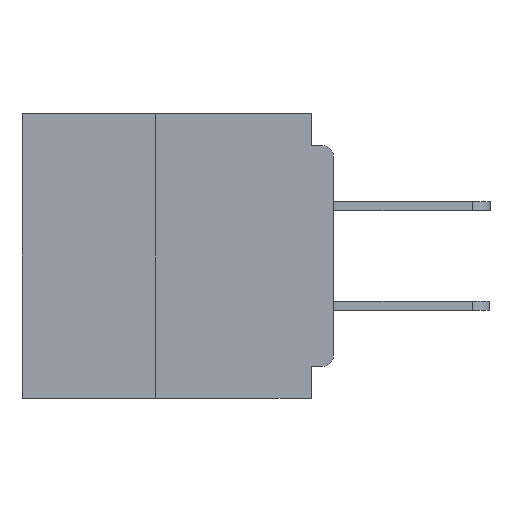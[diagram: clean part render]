
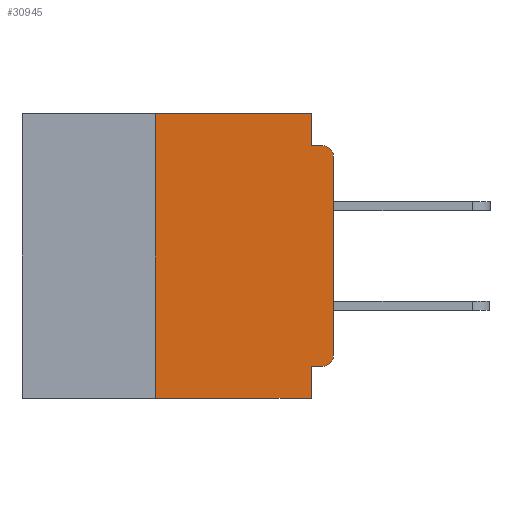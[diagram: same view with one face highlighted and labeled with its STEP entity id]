
A CAD part, left-side view. The second image highlights one B-rep face of the part: STEP entity #30945.
In plain terms, the highlighted planar face has unit normal (-1, 0, 0).
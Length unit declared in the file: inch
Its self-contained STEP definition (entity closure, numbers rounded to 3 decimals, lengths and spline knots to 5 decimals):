
#432 = VERTEX_POINT ( 'NONE', #10456 ) ;
#703 = VECTOR ( 'NONE', #32808, 39.37008 ) ;
#1035 = VECTOR ( 'NONE', #26939, 39.37008 ) ;
#1875 = ORIENTED_EDGE ( 'NONE', *, *, #35211, .T. ) ;
#3511 = ORIENTED_EDGE ( 'NONE', *, *, #10251, .F. ) ;
#3592 = DIRECTION ( 'NONE',  ( 1., 0., 0. ) ) ;
#3890 = LINE ( 'NONE', #31665, #19106 ) ;
#3931 = DIRECTION ( 'NONE',  ( 0., -1., 0. ) ) ;
#4588 = DIRECTION ( 'NONE',  ( 0., 1., 0. ) ) ;
#5513 = AXIS2_PLACEMENT_3D ( 'NONE', #20702, #3592, #23549 ) ;
#5674 = VECTOR ( 'NONE', #4588, 39.37008 ) ;
#6583 = VECTOR ( 'NONE', #20552, 39.37008 ) ;
#7860 = EDGE_CURVE ( 'NONE', #8786, #15277, #21474, .T. ) ;
#8786 = VERTEX_POINT ( 'NONE', #16869 ) ;
#8913 = VERTEX_POINT ( 'NONE', #28820 ) ;
#9740 = VECTOR ( 'NONE', #24982, 39.37008 ) ;
#9769 = VERTEX_POINT ( 'NONE', #35502 ) ;
#10196 = VERTEX_POINT ( 'NONE', #15524 ) ;
#10251 = EDGE_CURVE ( 'NONE', #12211, #9769, #30269, .T. ) ;
#10320 = EDGE_CURVE ( 'NONE', #432, #12211, #29380, .T. ) ;
#10379 = VECTOR ( 'NONE', #21185, 39.37008 ) ;
#10406 = CIRCLE ( 'NONE', #13544, 0.015 ) ;
#10456 = CARTESIAN_POINT ( 'NONE',  ( 0., 0.015, -0.355 ) ) ;
#10617 = LINE ( 'NONE', #36324, #9740 ) ;
#10820 = EDGE_CURVE ( 'NONE', #8913, #15277, #12352, .T. ) ;
#11535 = ORIENTED_EDGE ( 'NONE', *, *, #33857, .T. ) ;
#12211 = VERTEX_POINT ( 'NONE', #15884 ) ;
#12215 = VERTEX_POINT ( 'NONE', #18732 ) ;
#12264 = CARTESIAN_POINT ( 'NONE',  ( 0., 0.015, -0.06 ) ) ;
#12352 = LINE ( 'NONE', #23882, #19077 ) ;
#13316 = LINE ( 'NONE', #17721, #6583 ) ;
#13407 = DIRECTION ( 'NONE',  ( -1., 0., 0. ) ) ;
#13544 = AXIS2_PLACEMENT_3D ( 'NONE', #30482, #13407, #33330 ) ;
#14606 = DIRECTION ( 'NONE',  ( 0., -1., 0. ) ) ;
#15206 = DIRECTION ( 'NONE',  ( 0., 0., -1. ) ) ;
#15277 = VERTEX_POINT ( 'NONE', #33144 ) ;
#15524 = CARTESIAN_POINT ( 'NONE',  ( 0., 0.031, 0. ) ) ;
#15662 = CARTESIAN_POINT ( 'NONE',  ( 0., 0.031, 0. ) ) ;
#15858 = ORIENTED_EDGE ( 'NONE', *, *, #31444, .F. ) ;
#15884 = CARTESIAN_POINT ( 'NONE',  ( 0., 0.031, -0.355 ) ) ;
#16727 = AXIS2_PLACEMENT_3D ( 'NONE', #12264, #32255, #15206 ) ;
#16869 = CARTESIAN_POINT ( 'NONE',  ( 0., 0., -0.06 ) ) ;
#16980 = VERTEX_POINT ( 'NONE', #24636 ) ;
#17721 = CARTESIAN_POINT ( 'NONE',  ( 0., 0.25, -0.4 ) ) ;
#18043 = LINE ( 'NONE', #15662, #10379 ) ;
#18372 = CARTESIAN_POINT ( 'NONE',  ( 0., 0., 0. ) ) ;
#18519 = ORIENTED_EDGE ( 'NONE', *, *, #27547, .F. ) ;
#18553 = ORIENTED_EDGE ( 'NONE', *, *, #22475, .F. ) ;
#18732 = CARTESIAN_POINT ( 'NONE',  ( 0., 0., -0.34 ) ) ;
#19077 = VECTOR ( 'NONE', #3931, 39.37008 ) ;
#19106 = VECTOR ( 'NONE', #14606, 39.37008 ) ;
#20552 = DIRECTION ( 'NONE',  ( 0., 0., 1. ) ) ;
#20702 = CARTESIAN_POINT ( 'NONE',  ( 0., 0.437, 0. ) ) ;
#21185 = DIRECTION ( 'NONE',  ( 0., 0., -1. ) ) ;
#21474 = CIRCLE ( 'NONE', #16727, 0.015 ) ;
#22475 = EDGE_CURVE ( 'NONE', #16980, #10196, #10617, .T. ) ;
#22974 = ORIENTED_EDGE ( 'NONE', *, *, #10320, .F. ) ;
#23155 = EDGE_LOOP ( 'NONE', ( #1875, #34840, #28936, #18519, #18553, #15858, #11535, #3511, #22974, #29211 ) ) ;
#23549 = DIRECTION ( 'NONE',  ( 0., 0., -1. ) ) ;
#23882 = CARTESIAN_POINT ( 'NONE',  ( 0., 0., -0.045 ) ) ;
#24302 = CARTESIAN_POINT ( 'NONE',  ( 0., 0.031, -0.4 ) ) ;
#24636 = CARTESIAN_POINT ( 'NONE',  ( 0., 0.25, 0. ) ) ;
#24982 = DIRECTION ( 'NONE',  ( 0., -1., 0. ) ) ;
#25186 = EDGE_CURVE ( 'NONE', #432, #12215, #10406, .T. ) ;
#26939 = DIRECTION ( 'NONE',  ( 0., 0., 1. ) ) ;
#27547 = EDGE_CURVE ( 'NONE', #10196, #8913, #18043, .T. ) ;
#28820 = CARTESIAN_POINT ( 'NONE',  ( 0., 0.031, -0.045 ) ) ;
#28936 = ORIENTED_EDGE ( 'NONE', *, *, #10820, .F. ) ;
#29211 = ORIENTED_EDGE ( 'NONE', *, *, #25186, .T. ) ;
#29380 = LINE ( 'NONE', #33047, #5674 ) ;
#29426 = FACE_OUTER_BOUND ( 'NONE', #23155, .T. ) ;
#30269 = LINE ( 'NONE', #24302, #703 ) ;
#30482 = CARTESIAN_POINT ( 'NONE',  ( 0., 0.015, -0.34 ) ) ;
#30945 = ADVANCED_FACE ( 'NONE', ( #29426 ), #34846, .F. ) ;
#31444 = EDGE_CURVE ( 'NONE', #33290, #16980, #13316, .T. ) ;
#31665 = CARTESIAN_POINT ( 'NONE',  ( 0., 0.437, -0.4 ) ) ;
#32255 = DIRECTION ( 'NONE',  ( -1., 0., 0. ) ) ;
#32387 = LINE ( 'NONE', #18372, #1035 ) ;
#32808 = DIRECTION ( 'NONE',  ( 0., 0., -1. ) ) ;
#33047 = CARTESIAN_POINT ( 'NONE',  ( 0., 0., -0.355 ) ) ;
#33144 = CARTESIAN_POINT ( 'NONE',  ( 0., 0.015, -0.045 ) ) ;
#33290 = VERTEX_POINT ( 'NONE', #34459 ) ;
#33330 = DIRECTION ( 'NONE',  ( 0., 0., -1. ) ) ;
#33857 = EDGE_CURVE ( 'NONE', #33290, #9769, #3890, .T. ) ;
#34459 = CARTESIAN_POINT ( 'NONE',  ( 0., 0.25, -0.4 ) ) ;
#34840 = ORIENTED_EDGE ( 'NONE', *, *, #7860, .T. ) ;
#34846 = PLANE ( 'NONE',  #5513 ) ;
#35211 = EDGE_CURVE ( 'NONE', #12215, #8786, #32387, .T. ) ;
#35502 = CARTESIAN_POINT ( 'NONE',  ( 0., 0.031, -0.4 ) ) ;
#36324 = CARTESIAN_POINT ( 'NONE',  ( 0., 0.437, 0. ) ) ;
